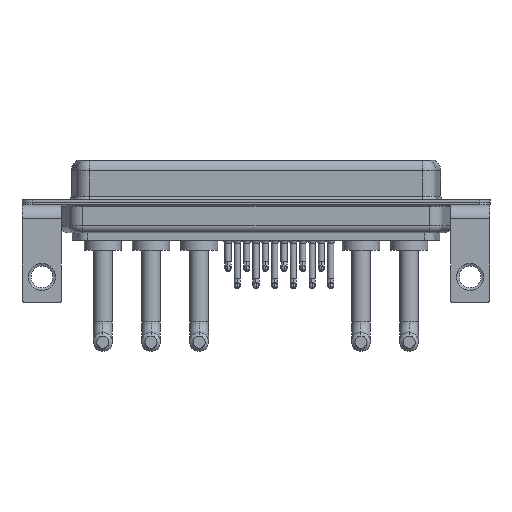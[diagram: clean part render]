
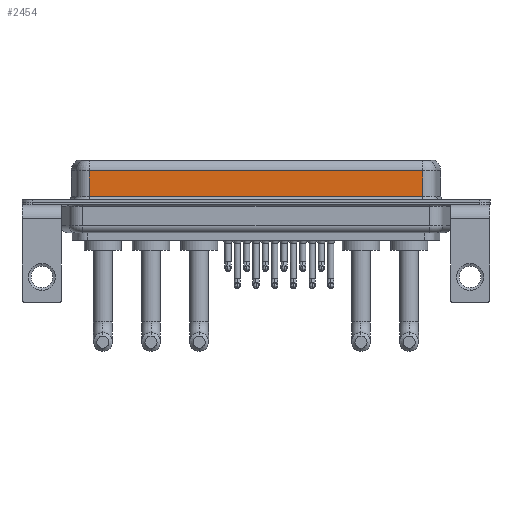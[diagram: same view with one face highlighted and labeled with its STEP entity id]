
A CAD part, front view. The second image highlights one B-rep face of the part: STEP entity #2454.
In plain terms, the highlighted planar face has unit normal (0, -1, 0).
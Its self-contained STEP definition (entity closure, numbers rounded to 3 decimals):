
#2041 = DIRECTION ( 'NONE',  ( 1., 0., 0. ) ) ;
#2385 = CARTESIAN_POINT ( 'NONE',  ( 7.038, -3.95, 6.4 ) ) ;
#2392 = DIRECTION ( 'NONE',  ( -1., 0., 0. ) ) ;
#2454 = ADVANCED_FACE ( 'NONE', ( #14783 ), #19525, .F. ) ;
#2719 = VERTEX_POINT ( 'NONE', #17794 ) ;
#4548 = ORIENTED_EDGE ( 'NONE', *, *, #13771, .T. ) ;
#5146 = DIRECTION ( 'NONE',  ( 0., 0., -1. ) ) ;
#5163 = VERTEX_POINT ( 'NONE', #17101 ) ;
#5695 = EDGE_CURVE ( 'NONE', #13654, #2719, #6643, .T. ) ;
#5774 = EDGE_CURVE ( 'NONE', #8823, #2719, #13241, .T. ) ;
#6643 = LINE ( 'NONE', #19764, #6984 ) ;
#6677 = VECTOR ( 'NONE', #5146, 1000. ) ;
#6984 = VECTOR ( 'NONE', #2041, 1000. ) ;
#8097 = DIRECTION ( 'NONE',  ( 0., 1., 0. ) ) ;
#8823 = VERTEX_POINT ( 'NONE', #18833 ) ;
#9234 = VECTOR ( 'NONE', #2392, 1000. ) ;
#10867 = EDGE_LOOP ( 'NONE', ( #11933, #15246, #4548, #20268 ) ) ;
#11933 = ORIENTED_EDGE ( 'NONE', *, *, #5774, .F. ) ;
#13154 = CARTESIAN_POINT ( 'NONE',  ( 7.038, -3.95, 0.9 ) ) ;
#13241 = LINE ( 'NONE', #19659, #6677 ) ;
#13654 = VERTEX_POINT ( 'NONE', #13154 ) ;
#13771 = EDGE_CURVE ( 'NONE', #5163, #13654, #16950, .T. ) ;
#14783 = FACE_OUTER_BOUND ( 'NONE', #10867, .T. ) ;
#15246 = ORIENTED_EDGE ( 'NONE', *, *, #18012, .T. ) ;
#15373 = DIRECTION ( 'NONE',  ( 0., 0., -1. ) ) ;
#15783 = AXIS2_PLACEMENT_3D ( 'NONE', #19618, #8097, #18034 ) ;
#16950 = LINE ( 'NONE', #2385, #20572 ) ;
#16956 = LINE ( 'NONE', #19791, #9234 ) ;
#17101 = CARTESIAN_POINT ( 'NONE',  ( 7.038, -3.95, 4.65 ) ) ;
#17794 = CARTESIAN_POINT ( 'NONE',  ( 56.462, -3.95, 0.9 ) ) ;
#18012 = EDGE_CURVE ( 'NONE', #8823, #5163, #16956, .T. ) ;
#18034 = DIRECTION ( 'NONE',  ( 0., 0., 1. ) ) ;
#18833 = CARTESIAN_POINT ( 'NONE',  ( 56.462, -3.95, 4.65 ) ) ;
#19525 = PLANE ( 'NONE',  #15783 ) ;
#19618 = CARTESIAN_POINT ( 'NONE',  ( 56.462, -3.95, 6.4 ) ) ;
#19659 = CARTESIAN_POINT ( 'NONE',  ( 56.462, -3.95, 6.4 ) ) ;
#19764 = CARTESIAN_POINT ( 'NONE',  ( 56.462, -3.95, 0.9 ) ) ;
#19791 = CARTESIAN_POINT ( 'NONE',  ( 56.462, -3.95, 4.65 ) ) ;
#20268 = ORIENTED_EDGE ( 'NONE', *, *, #5695, .T. ) ;
#20572 = VECTOR ( 'NONE', #15373, 1000. ) ;
